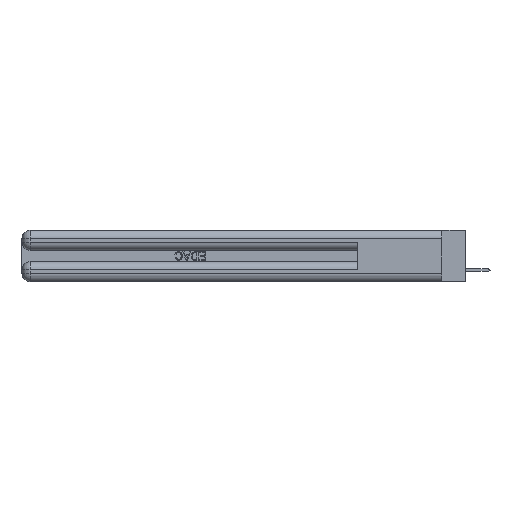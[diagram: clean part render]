
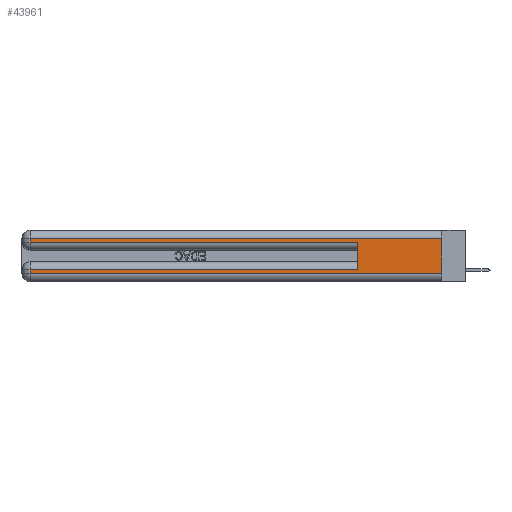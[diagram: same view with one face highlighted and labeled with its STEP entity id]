
A CAD part, left-side view. The second image highlights one B-rep face of the part: STEP entity #43961.
In plain terms, the highlighted planar face has unit normal (-1, 0, 0).
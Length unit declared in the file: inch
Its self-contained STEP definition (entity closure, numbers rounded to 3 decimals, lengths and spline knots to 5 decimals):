
#563 = EDGE_CURVE ( 'NONE', #45671, #43375, #14540, .T. ) ;
#1396 = LINE ( 'NONE', #42540, #17273 ) ;
#2084 = CARTESIAN_POINT ( 'NONE',  ( 0., 2.94, 0.37 ) ) ;
#2397 = ORIENTED_EDGE ( 'NONE', *, *, #39384, .T. ) ;
#3717 = DIRECTION ( 'NONE',  ( 1., 0., 0. ) ) ;
#4132 = EDGE_CURVE ( 'NONE', #35200, #29878, #1396, .T. ) ;
#4247 = CARTESIAN_POINT ( 'NONE',  ( 0., 0., 0.085 ) ) ;
#4366 = CARTESIAN_POINT ( 'NONE',  ( 0., 0., 0.06 ) ) ;
#7775 = VECTOR ( 'NONE', #34068, 39.37008 ) ;
#7819 = VERTEX_POINT ( 'NONE', #36627 ) ;
#8327 = DIRECTION ( 'NONE',  ( 0., 1., 0. ) ) ;
#9200 = ORIENTED_EDGE ( 'NONE', *, *, #16978, .T. ) ;
#9943 = DIRECTION ( 'NONE',  ( 0., 0., 1. ) ) ;
#10608 = CARTESIAN_POINT ( 'NONE',  ( 0., 0.6, 0.085 ) ) ;
#10948 = ORIENTED_EDGE ( 'NONE', *, *, #27361, .T. ) ;
#11467 = CARTESIAN_POINT ( 'NONE',  ( 0., 2.94, 0.285 ) ) ;
#12058 = CARTESIAN_POINT ( 'NONE',  ( 0., 0., 0.37 ) ) ;
#13077 = CARTESIAN_POINT ( 'NONE',  ( 0., 0.6, 0.285 ) ) ;
#14540 = LINE ( 'NONE', #4247, #17021 ) ;
#14714 = CARTESIAN_POINT ( 'NONE',  ( 0., 0., 0.31 ) ) ;
#15651 = DIRECTION ( 'NONE',  ( 0., 0., -1. ) ) ;
#16978 = EDGE_CURVE ( 'NONE', #29878, #32937, #39501, .T. ) ;
#17021 = VECTOR ( 'NONE', #8327, 39.37008 ) ;
#17273 = VECTOR ( 'NONE', #50902, 39.37008 ) ;
#17382 = VECTOR ( 'NONE', #25396, 39.37008 ) ;
#18445 = LINE ( 'NONE', #12058, #20944 ) ;
#18914 = VERTEX_POINT ( 'NONE', #14714 ) ;
#20371 = CARTESIAN_POINT ( 'NONE',  ( 0., 0., 0.37 ) ) ;
#20944 = VECTOR ( 'NONE', #15651, 39.37008 ) ;
#21568 = AXIS2_PLACEMENT_3D ( 'NONE', #20371, #3717, #48659 ) ;
#22015 = VERTEX_POINT ( 'NONE', #27261 ) ;
#25396 = DIRECTION ( 'NONE',  ( 0., 1., 0. ) ) ;
#26053 = CARTESIAN_POINT ( 'NONE',  ( 0., 0.6, 0.145 ) ) ;
#26255 = VECTOR ( 'NONE', #9943, 39.37008 ) ;
#27261 = CARTESIAN_POINT ( 'NONE',  ( 0., 2.94, 0.06 ) ) ;
#27361 = EDGE_CURVE ( 'NONE', #18914, #35200, #36411, .T. ) ;
#27535 = VECTOR ( 'NONE', #30075, 39.37008 ) ;
#27549 = LINE ( 'NONE', #26053, #26255 ) ;
#28714 = ORIENTED_EDGE ( 'NONE', *, *, #4132, .T. ) ;
#29815 = CARTESIAN_POINT ( 'NONE',  ( 0., 0., 0.285 ) ) ;
#29878 = VERTEX_POINT ( 'NONE', #11467 ) ;
#30075 = DIRECTION ( 'NONE',  ( 0., 0., -1. ) ) ;
#31430 = FACE_OUTER_BOUND ( 'NONE', #48354, .T. ) ;
#32712 = ORIENTED_EDGE ( 'NONE', *, *, #46836, .T. ) ;
#32937 = VERTEX_POINT ( 'NONE', #13077 ) ;
#33329 = LINE ( 'NONE', #4366, #48547 ) ;
#34068 = DIRECTION ( 'NONE',  ( 0., -1., 0. ) ) ;
#35200 = VERTEX_POINT ( 'NONE', #40272 ) ;
#36411 = LINE ( 'NONE', #40979, #17382 ) ;
#36627 = CARTESIAN_POINT ( 'NONE',  ( 0., 0., 0.06 ) ) ;
#36636 = ORIENTED_EDGE ( 'NONE', *, *, #41019, .F. ) ;
#39384 = EDGE_CURVE ( 'NONE', #43375, #22015, #49009, .T. ) ;
#39501 = LINE ( 'NONE', #29815, #7775 ) ;
#40272 = CARTESIAN_POINT ( 'NONE',  ( 0., 2.94, 0.31 ) ) ;
#40979 = CARTESIAN_POINT ( 'NONE',  ( 0., 0., 0.31 ) ) ;
#41019 = EDGE_CURVE ( 'NONE', #18914, #7819, #18445, .T. ) ;
#42540 = CARTESIAN_POINT ( 'NONE',  ( 0., 2.94, 0.37 ) ) ;
#42765 = ORIENTED_EDGE ( 'NONE', *, *, #563, .T. ) ;
#43375 = VERTEX_POINT ( 'NONE', #51769 ) ;
#43961 = ADVANCED_FACE ( 'NONE', ( #31430 ), #44553, .F. ) ;
#44553 = PLANE ( 'NONE',  #21568 ) ;
#45004 = EDGE_CURVE ( 'NONE', #45671, #32937, #27549, .T. ) ;
#45023 = ORIENTED_EDGE ( 'NONE', *, *, #45004, .F. ) ;
#45671 = VERTEX_POINT ( 'NONE', #10608 ) ;
#46836 = EDGE_CURVE ( 'NONE', #22015, #7819, #33329, .T. ) ;
#48354 = EDGE_LOOP ( 'NONE', ( #36636, #10948, #28714, #9200, #45023, #42765, #2397, #32712 ) ) ;
#48547 = VECTOR ( 'NONE', #49500, 39.37008 ) ;
#48659 = DIRECTION ( 'NONE',  ( 0., 0., -1. ) ) ;
#49009 = LINE ( 'NONE', #2084, #27535 ) ;
#49500 = DIRECTION ( 'NONE',  ( 0., -1., 0. ) ) ;
#50902 = DIRECTION ( 'NONE',  ( 0., 0., -1. ) ) ;
#51769 = CARTESIAN_POINT ( 'NONE',  ( 0., 2.94, 0.085 ) ) ;
